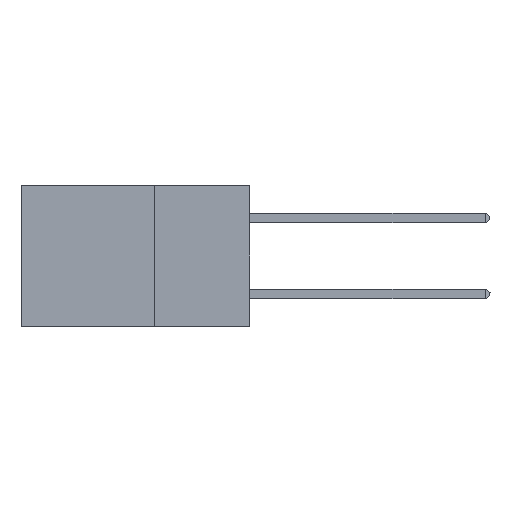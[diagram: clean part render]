
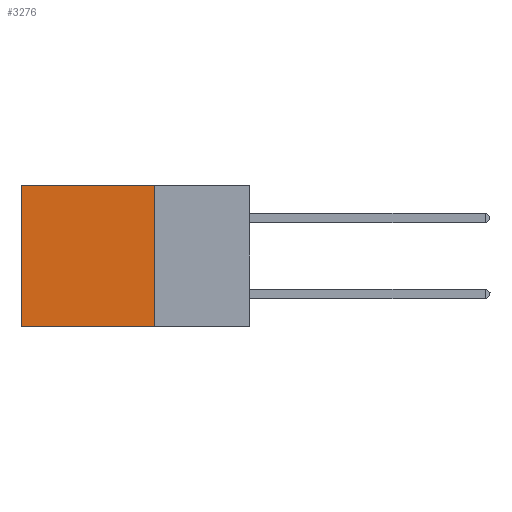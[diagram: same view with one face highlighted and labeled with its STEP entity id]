
A CAD part, left-side view. The second image highlights one B-rep face of the part: STEP entity #3276.
In plain terms, the highlighted planar face has unit normal (-1, 0, 0).
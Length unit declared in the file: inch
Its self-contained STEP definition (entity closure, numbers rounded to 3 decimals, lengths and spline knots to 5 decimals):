
#3276 = ADVANCED_FACE ( 'NONE', ( #4799 ), #38176, .F. ) ;
#4118 = LINE ( 'NONE', #11460, #17371 ) ;
#4201 = DIRECTION ( 'NONE',  ( 0., 1., 0. ) ) ;
#4682 = VERTEX_POINT ( 'NONE', #33394 ) ;
#4780 = CARTESIAN_POINT ( 'NONE',  ( 0.2875, 0.25, 0. ) ) ;
#4799 = FACE_OUTER_BOUND ( 'NONE', #36441, .T. ) ;
#5878 = ORIENTED_EDGE ( 'NONE', *, *, #43325, .F. ) ;
#7506 = EDGE_CURVE ( 'NONE', #28826, #9917, #30308, .T. ) ;
#8016 = DIRECTION ( 'NONE',  ( 1., 0., 0. ) ) ;
#8470 = LINE ( 'NONE', #17722, #40868 ) ;
#9917 = VERTEX_POINT ( 'NONE', #11936 ) ;
#10839 = VERTEX_POINT ( 'NONE', #13540 ) ;
#11460 = CARTESIAN_POINT ( 'NONE',  ( 0.2875, 0.25, -0.37 ) ) ;
#11936 = CARTESIAN_POINT ( 'NONE',  ( 0.2875, 0.6, 0. ) ) ;
#12559 = DIRECTION ( 'NONE',  ( 0., 1., 0. ) ) ;
#12624 = LINE ( 'NONE', #38409, #39658 ) ;
#13540 = CARTESIAN_POINT ( 'NONE',  ( 0.2875, 0.25, -0.37 ) ) ;
#15189 = AXIS2_PLACEMENT_3D ( 'NONE', #4780, #8016, #17832 ) ;
#15499 = EDGE_CURVE ( 'NONE', #28826, #10839, #8470, .T. ) ;
#15797 = CARTESIAN_POINT ( 'NONE',  ( 0.2875, 0.25, 0. ) ) ;
#17051 = EDGE_CURVE ( 'NONE', #9917, #4682, #12624, .T. ) ;
#17371 = VECTOR ( 'NONE', #4201, 39.37008 ) ;
#17722 = CARTESIAN_POINT ( 'NONE',  ( 0.2875, 0.25, 0. ) ) ;
#17772 = ORIENTED_EDGE ( 'NONE', *, *, #15499, .F. ) ;
#17832 = DIRECTION ( 'NONE',  ( 0., 0., -1. ) ) ;
#18072 = DIRECTION ( 'NONE',  ( 0., 0., -1. ) ) ;
#18166 = DIRECTION ( 'NONE',  ( 0., 0., -1. ) ) ;
#21265 = VECTOR ( 'NONE', #12559, 39.37008 ) ;
#25327 = ORIENTED_EDGE ( 'NONE', *, *, #17051, .T. ) ;
#28826 = VERTEX_POINT ( 'NONE', #36784 ) ;
#30308 = LINE ( 'NONE', #15797, #21265 ) ;
#33394 = CARTESIAN_POINT ( 'NONE',  ( 0.2875, 0.6, -0.37 ) ) ;
#36441 = EDGE_LOOP ( 'NONE', ( #25327, #5878, #17772, #43075 ) ) ;
#36784 = CARTESIAN_POINT ( 'NONE',  ( 0.2875, 0.25, 0. ) ) ;
#38176 = PLANE ( 'NONE',  #15189 ) ;
#38409 = CARTESIAN_POINT ( 'NONE',  ( 0.2875, 0.6, 0. ) ) ;
#39658 = VECTOR ( 'NONE', #18072, 39.37008 ) ;
#40868 = VECTOR ( 'NONE', #18166, 39.37008 ) ;
#43075 = ORIENTED_EDGE ( 'NONE', *, *, #7506, .T. ) ;
#43325 = EDGE_CURVE ( 'NONE', #10839, #4682, #4118, .T. ) ;
